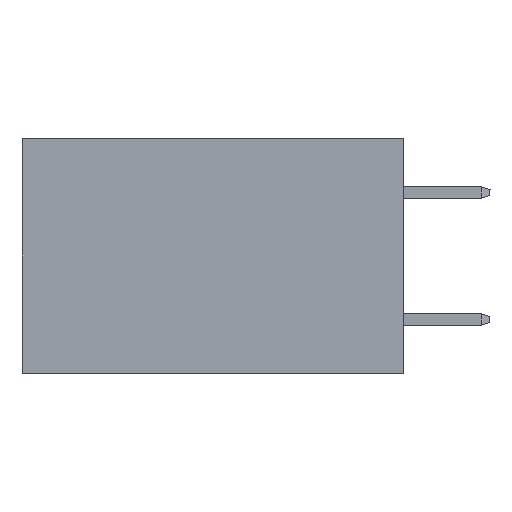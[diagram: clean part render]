
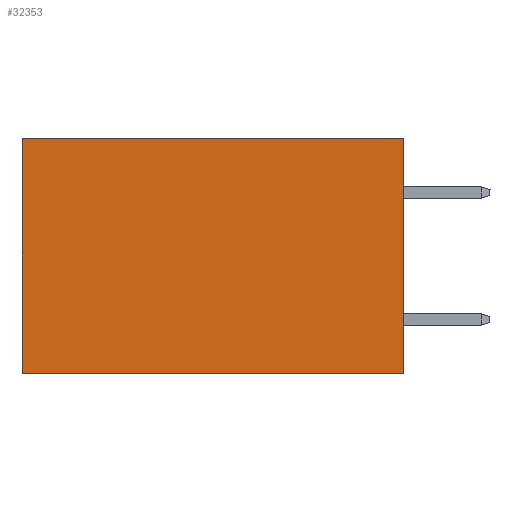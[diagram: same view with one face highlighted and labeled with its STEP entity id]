
A CAD part, left-side view. The second image highlights one B-rep face of the part: STEP entity #32353.
In plain terms, the highlighted planar face has unit normal (-1, 0, 0).
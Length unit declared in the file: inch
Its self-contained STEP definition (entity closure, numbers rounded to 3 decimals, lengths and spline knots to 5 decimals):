
#204 = CARTESIAN_POINT ( 'NONE',  ( 0.2875, 0., 0. ) ) ;
#1201 = EDGE_CURVE ( 'NONE', #7440, #26802, #8567, .T. ) ;
#2163 = CARTESIAN_POINT ( 'NONE',  ( 0.2875, 0., 0. ) ) ;
#2169 = DIRECTION ( 'NONE',  ( 0., 0., -1. ) ) ;
#4823 = VECTOR ( 'NONE', #40406, 39.37008 ) ;
#5006 = DIRECTION ( 'NONE',  ( 0., 0., -1. ) ) ;
#6604 = PLANE ( 'NONE',  #23710 ) ;
#7440 = VERTEX_POINT ( 'NONE', #40755 ) ;
#7472 = DIRECTION ( 'NONE',  ( 0., 1., 0. ) ) ;
#8340 = LINE ( 'NONE', #37876, #26557 ) ;
#8567 = LINE ( 'NONE', #32548, #32929 ) ;
#9302 = VERTEX_POINT ( 'NONE', #31614 ) ;
#10154 = DIRECTION ( 'NONE',  ( 0., 0., -1. ) ) ;
#11448 = EDGE_CURVE ( 'NONE', #26802, #9302, #8340, .T. ) ;
#15438 = VECTOR ( 'NONE', #2169, 39.37008 ) ;
#15691 = LINE ( 'NONE', #42559, #15438 ) ;
#19164 = CARTESIAN_POINT ( 'NONE',  ( 0.2875, 0.6, 0. ) ) ;
#19829 = ORIENTED_EDGE ( 'NONE', *, *, #40931, .T. ) ;
#22251 = ORIENTED_EDGE ( 'NONE', *, *, #1201, .F. ) ;
#23710 = AXIS2_PLACEMENT_3D ( 'NONE', #2163, #30808, #10154 ) ;
#26455 = LINE ( 'NONE', #204, #4823 ) ;
#26557 = VECTOR ( 'NONE', #7472, 39.37008 ) ;
#26802 = VERTEX_POINT ( 'NONE', #35609 ) ;
#26831 = FACE_OUTER_BOUND ( 'NONE', #34877, .T. ) ;
#28387 = VERTEX_POINT ( 'NONE', #19164 ) ;
#30808 = DIRECTION ( 'NONE',  ( 1., 0., 0. ) ) ;
#31059 = ORIENTED_EDGE ( 'NONE', *, *, #40704, .T. ) ;
#31614 = CARTESIAN_POINT ( 'NONE',  ( 0.2875, 0.6, -0.37 ) ) ;
#32165 = ORIENTED_EDGE ( 'NONE', *, *, #11448, .F. ) ;
#32353 = ADVANCED_FACE ( 'NONE', ( #26831 ), #6604, .F. ) ;
#32548 = CARTESIAN_POINT ( 'NONE',  ( 0.2875, 0., 0. ) ) ;
#32929 = VECTOR ( 'NONE', #5006, 39.37008 ) ;
#34877 = EDGE_LOOP ( 'NONE', ( #19829, #32165, #22251, #31059 ) ) ;
#35609 = CARTESIAN_POINT ( 'NONE',  ( 0.2875, 0., -0.37 ) ) ;
#37876 = CARTESIAN_POINT ( 'NONE',  ( 0.2875, 0., -0.37 ) ) ;
#40406 = DIRECTION ( 'NONE',  ( 0., 1., 0. ) ) ;
#40704 = EDGE_CURVE ( 'NONE', #7440, #28387, #26455, .T. ) ;
#40755 = CARTESIAN_POINT ( 'NONE',  ( 0.2875, 0., 0. ) ) ;
#40931 = EDGE_CURVE ( 'NONE', #28387, #9302, #15691, .T. ) ;
#42559 = CARTESIAN_POINT ( 'NONE',  ( 0.2875, 0.6, 0. ) ) ;
